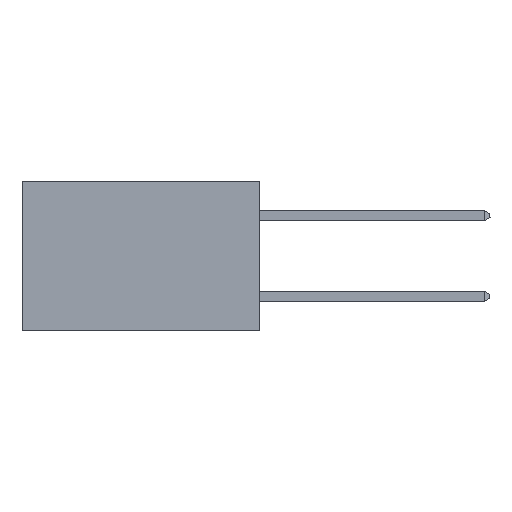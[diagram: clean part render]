
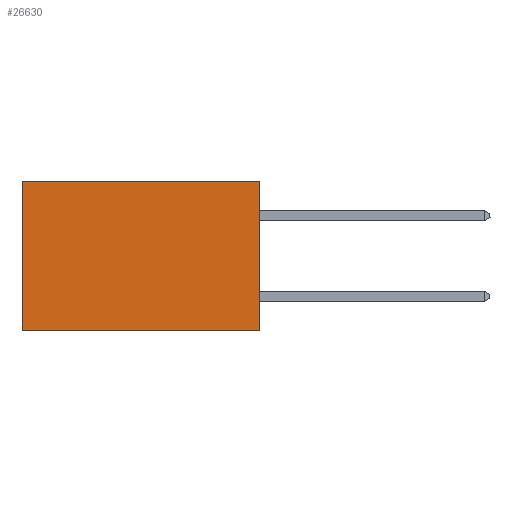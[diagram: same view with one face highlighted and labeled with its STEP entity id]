
A CAD part, left-side view. The second image highlights one B-rep face of the part: STEP entity #26630.
In plain terms, the highlighted planar face has unit normal (-1, 0, 0).
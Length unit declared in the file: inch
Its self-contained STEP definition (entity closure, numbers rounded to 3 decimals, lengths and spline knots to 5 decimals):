
#224 = CARTESIAN_POINT ( 'NONE',  ( 0.277, 0.59, 0. ) ) ;
#365 = DIRECTION ( 'NONE',  ( 0., 1., 0. ) ) ;
#1258 = LINE ( 'NONE', #19906, #11165 ) ;
#1646 = LINE ( 'NONE', #15239, #17178 ) ;
#3821 = LINE ( 'NONE', #16689, #26114 ) ;
#4773 = ORIENTED_EDGE ( 'NONE', *, *, #26650, .F. ) ;
#4939 = ORIENTED_EDGE ( 'NONE', *, *, #19051, .F. ) ;
#5986 = VECTOR ( 'NONE', #14962, 39.37008 ) ;
#6035 = ORIENTED_EDGE ( 'NONE', *, *, #14464, .T. ) ;
#6835 = CARTESIAN_POINT ( 'NONE',  ( 0.277, 0.59, -0.37 ) ) ;
#8869 = ORIENTED_EDGE ( 'NONE', *, *, #25118, .T. ) ;
#10302 = CARTESIAN_POINT ( 'NONE',  ( 0.277, 0., -0.37 ) ) ;
#10681 = VERTEX_POINT ( 'NONE', #12190 ) ;
#10803 = CARTESIAN_POINT ( 'NONE',  ( 0.277, 0., 0. ) ) ;
#11165 = VECTOR ( 'NONE', #13597, 39.37008 ) ;
#11209 = EDGE_LOOP ( 'NONE', ( #8869, #4939, #4773, #6035 ) ) ;
#12190 = CARTESIAN_POINT ( 'NONE',  ( 0.277, 0., -0.37 ) ) ;
#12434 = DIRECTION ( 'NONE',  ( 1., 0., 0. ) ) ;
#13597 = DIRECTION ( 'NONE',  ( 0., 0., -1. ) ) ;
#14464 = EDGE_CURVE ( 'NONE', #16889, #24793, #15217, .T. ) ;
#14962 = DIRECTION ( 'NONE',  ( 0., 1., 0. ) ) ;
#15018 = FACE_OUTER_BOUND ( 'NONE', #11209, .T. ) ;
#15159 = CARTESIAN_POINT ( 'NONE',  ( 0.277, 0., 0. ) ) ;
#15217 = LINE ( 'NONE', #10803, #5986 ) ;
#15239 = CARTESIAN_POINT ( 'NONE',  ( 0.277, 0., -0.37 ) ) ;
#15621 = VERTEX_POINT ( 'NONE', #6835 ) ;
#16689 = CARTESIAN_POINT ( 'NONE',  ( 0.277, 0., -0.37 ) ) ;
#16889 = VERTEX_POINT ( 'NONE', #15159 ) ;
#17178 = VECTOR ( 'NONE', #365, 39.37008 ) ;
#19051 = EDGE_CURVE ( 'NONE', #10681, #15621, #1646, .T. ) ;
#19906 = CARTESIAN_POINT ( 'NONE',  ( 0.277, 0.59, -0.37 ) ) ;
#20949 = DIRECTION ( 'NONE',  ( 0., 0., -1. ) ) ;
#22919 = PLANE ( 'NONE',  #24770 ) ;
#24770 = AXIS2_PLACEMENT_3D ( 'NONE', #10302, #12434, #27018 ) ;
#24793 = VERTEX_POINT ( 'NONE', #224 ) ;
#25118 = EDGE_CURVE ( 'NONE', #24793, #15621, #1258, .T. ) ;
#26114 = VECTOR ( 'NONE', #20949, 39.37008 ) ;
#26630 = ADVANCED_FACE ( 'NONE', ( #15018 ), #22919, .F. ) ;
#26650 = EDGE_CURVE ( 'NONE', #16889, #10681, #3821, .T. ) ;
#27018 = DIRECTION ( 'NONE',  ( 0., 0., -1. ) ) ;
